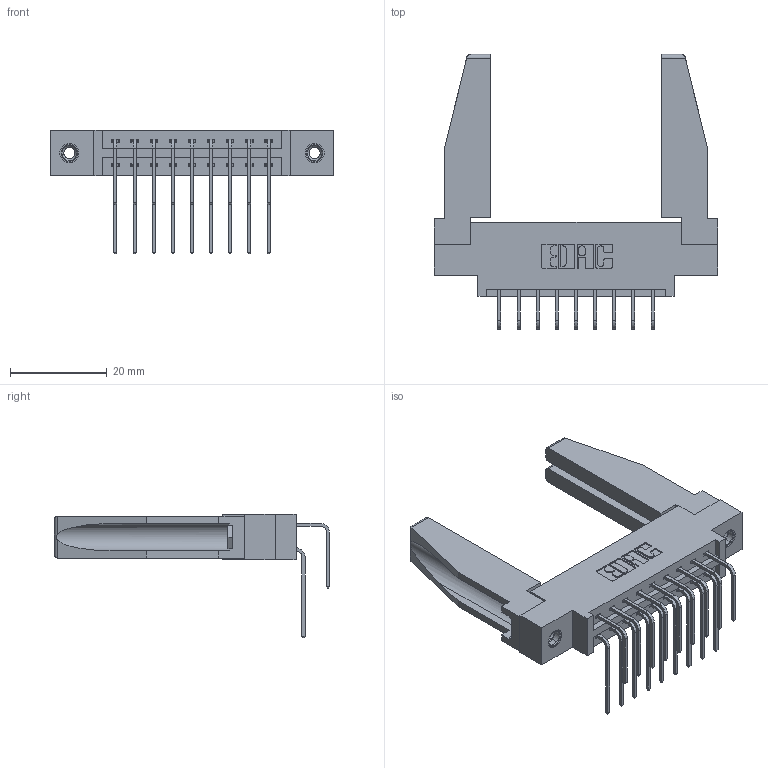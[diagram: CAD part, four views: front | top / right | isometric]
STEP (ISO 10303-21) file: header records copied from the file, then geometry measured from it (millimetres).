
FILE_DESCRIPTION (( 'STEP AP203' ), '1' );
FILE_NAME ('337-018-558-878.STEP', '2019-10-10T18:59:56', ( '' ), ( '' ), 'SwSTEP 2.0', 'SolidWorks 2016', '' );
FILE_SCHEMA (( 'CONFIG_CONTROL_DESIGN' ));
Length unit declared in the file: inch
Products named in the file (6): 345-292-001_558 Tail - 2; 337 Part_0.170 Offset - 0.156 Dia-TI; 345-292-001_558 559 Tail - 1; 345-250-001_345-250-001-102; 307-220-078; 337-018-558-878
Assembly tree (23 placements, depth 2):
  337-018-558-878
    337 Part_0.170 Offset - 0.156 Dia-TI
    345-292-001_558 559 Tail - 1  x9
    345-292-001_558 Tail - 2  x9
    345-250-001_345-250-001-102  x2
    307-220-078  x2
Bounding box: 58.67 x 56.96 x 25.53 mm (x, y, z)
Volume: 9723.9 mm3; surface area: 10617.6 mm2
Topology: 23 solids, 23 shells, 1256 faces, 3659 edges, 2406 vertices
Faces by surface type: plane 878, cylinder 362, cone 12, torus 4
Entity records: 15602 total; most frequent: CARTESIAN_POINT 2703, ORIENTED_EDGE 2544, DIRECTION 2348, EDGE_CURVE 1272, VECTOR 1066, LINE 1066, VERTEX_POINT 840, AXIS2_PLACEMENT_3D 641
